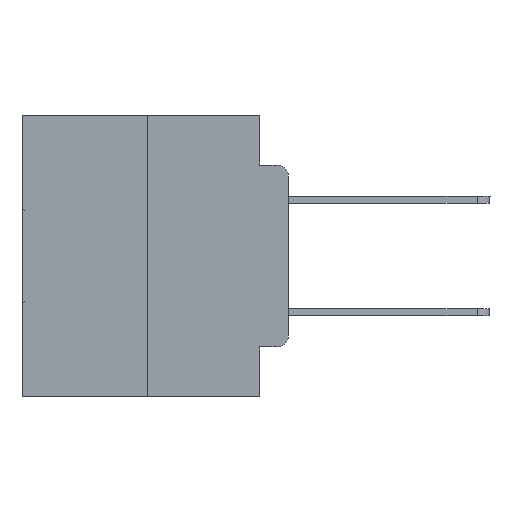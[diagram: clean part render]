
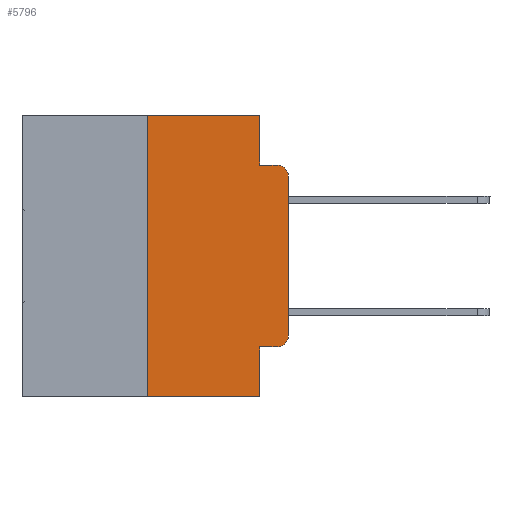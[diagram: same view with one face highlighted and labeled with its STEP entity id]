
A CAD part, left-side view. The second image highlights one B-rep face of the part: STEP entity #5796.
In plain terms, the highlighted planar face has unit normal (-1, 0, 0).
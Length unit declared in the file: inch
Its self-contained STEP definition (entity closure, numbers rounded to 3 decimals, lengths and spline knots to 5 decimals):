
#1228 = LINE ( 'NONE', #22122, #13435 ) ;
#1275 = CARTESIAN_POINT ( 'NONE',  ( 0., 0.051, -0.4115 ) ) ;
#1352 = DIRECTION ( 'NONE',  ( -1., 0., 0. ) ) ;
#1853 = VECTOR ( 'NONE', #12058, 39.37008 ) ;
#3068 = LINE ( 'NONE', #18056, #27924 ) ;
#3337 = ORIENTED_EDGE ( 'NONE', *, *, #27171, .F. ) ;
#3421 = AXIS2_PLACEMENT_3D ( 'NONE', #15892, #1352, #18319 ) ;
#3536 = DIRECTION ( 'NONE',  ( 0., -1., 0. ) ) ;
#3930 = DIRECTION ( 'NONE',  ( 0., -1., 0. ) ) ;
#3946 = CARTESIAN_POINT ( 'NONE',  ( 0., 0., -0.3915 ) ) ;
#3960 = LINE ( 'NONE', #30755, #26572 ) ;
#3976 = EDGE_CURVE ( 'NONE', #16938, #4100, #16561, .T. ) ;
#4100 = VERTEX_POINT ( 'NONE', #24785 ) ;
#4166 = AXIS2_PLACEMENT_3D ( 'NONE', #12298, #22362, #8027 ) ;
#4301 = CARTESIAN_POINT ( 'NONE',  ( 0., 0.051, -0.5 ) ) ;
#4887 = ORIENTED_EDGE ( 'NONE', *, *, #30881, .T. ) ;
#5540 = PLANE ( 'NONE',  #4166 ) ;
#5641 = EDGE_CURVE ( 'NONE', #4100, #10198, #3960, .T. ) ;
#5796 = ADVANCED_FACE ( 'NONE', ( #29119 ), #5540, .F. ) ;
#6980 = VECTOR ( 'NONE', #19574, 39.37008 ) ;
#7313 = EDGE_CURVE ( 'NONE', #11000, #10198, #14852, .T. ) ;
#7492 = VERTEX_POINT ( 'NONE', #21331 ) ;
#7603 = ORIENTED_EDGE ( 'NONE', *, *, #3976, .F. ) ;
#7668 = CIRCLE ( 'NONE', #25949, 0.02 ) ;
#7752 = LINE ( 'NONE', #17192, #6980 ) ;
#8027 = DIRECTION ( 'NONE',  ( 0., 0., -1. ) ) ;
#8768 = EDGE_CURVE ( 'NONE', #22448, #11916, #16369, .T. ) ;
#9472 = VECTOR ( 'NONE', #16045, 39.37008 ) ;
#9676 = CARTESIAN_POINT ( 'NONE',  ( 0., 0., 0. ) ) ;
#10119 = VERTEX_POINT ( 'NONE', #13116 ) ;
#10131 = EDGE_CURVE ( 'NONE', #10119, #16938, #3068, .T. ) ;
#10198 = VERTEX_POINT ( 'NONE', #25469 ) ;
#11000 = VERTEX_POINT ( 'NONE', #29747 ) ;
#11916 = VERTEX_POINT ( 'NONE', #4301 ) ;
#12058 = DIRECTION ( 'NONE',  ( 0., 0., 1. ) ) ;
#12298 = CARTESIAN_POINT ( 'NONE',  ( 0., 0.473, 0. ) ) ;
#12452 = ORIENTED_EDGE ( 'NONE', *, *, #5641, .F. ) ;
#13116 = CARTESIAN_POINT ( 'NONE',  ( 0., 0.25, 0. ) ) ;
#13325 = EDGE_CURVE ( 'NONE', #7492, #24728, #7668, .T. ) ;
#13435 = VECTOR ( 'NONE', #24535, 39.37008 ) ;
#13607 = CARTESIAN_POINT ( 'NONE',  ( 0., 0.051, -0.4115 ) ) ;
#13748 = EDGE_CURVE ( 'NONE', #24728, #11000, #14777, .T. ) ;
#14398 = CARTESIAN_POINT ( 'NONE',  ( 0., 0.02, -0.3915 ) ) ;
#14777 = LINE ( 'NONE', #9676, #1853 ) ;
#14852 = CIRCLE ( 'NONE', #3421, 0.02 ) ;
#15745 = CARTESIAN_POINT ( 'NONE',  ( 0., 0.051, 0. ) ) ;
#15892 = CARTESIAN_POINT ( 'NONE',  ( 0., 0.02, -0.1085 ) ) ;
#16045 = DIRECTION ( 'NONE',  ( 0., 0., -1. ) ) ;
#16111 = CARTESIAN_POINT ( 'NONE',  ( 0., 0.051, 0. ) ) ;
#16369 = LINE ( 'NONE', #22508, #21995 ) ;
#16561 = LINE ( 'NONE', #16111, #9472 ) ;
#16798 = EDGE_LOOP ( 'NONE', ( #29998, #24460, #12452, #7603, #26714, #21093, #28191, #3337, #4887, #18168 ) ) ;
#16825 = DIRECTION ( 'NONE',  ( 0., 0., -1. ) ) ;
#16938 = VERTEX_POINT ( 'NONE', #15745 ) ;
#17192 = CARTESIAN_POINT ( 'NONE',  ( 0., 0.25, 0. ) ) ;
#18056 = CARTESIAN_POINT ( 'NONE',  ( 0., 0.473, 0. ) ) ;
#18168 = ORIENTED_EDGE ( 'NONE', *, *, #13325, .T. ) ;
#18319 = DIRECTION ( 'NONE',  ( 0., 0., -1. ) ) ;
#19028 = CARTESIAN_POINT ( 'NONE',  ( 0., 0.25, -0.5 ) ) ;
#19574 = DIRECTION ( 'NONE',  ( 0., 0., 1. ) ) ;
#19837 = VERTEX_POINT ( 'NONE', #1275 ) ;
#20094 = DIRECTION ( 'NONE',  ( 0., -1., 0. ) ) ;
#21093 = ORIENTED_EDGE ( 'NONE', *, *, #28740, .F. ) ;
#21331 = CARTESIAN_POINT ( 'NONE',  ( 0., 0.02, -0.4115 ) ) ;
#21995 = VECTOR ( 'NONE', #20094, 39.37008 ) ;
#22122 = CARTESIAN_POINT ( 'NONE',  ( 0., 0.051, 0. ) ) ;
#22362 = DIRECTION ( 'NONE',  ( 1., 0., 0. ) ) ;
#22448 = VERTEX_POINT ( 'NONE', #19028 ) ;
#22508 = CARTESIAN_POINT ( 'NONE',  ( 0., 0.473, -0.5 ) ) ;
#24460 = ORIENTED_EDGE ( 'NONE', *, *, #7313, .T. ) ;
#24535 = DIRECTION ( 'NONE',  ( 0., 0., -1. ) ) ;
#24728 = VERTEX_POINT ( 'NONE', #3946 ) ;
#24785 = CARTESIAN_POINT ( 'NONE',  ( 0., 0.051, -0.0885 ) ) ;
#25212 = VECTOR ( 'NONE', #3930, 39.37008 ) ;
#25469 = CARTESIAN_POINT ( 'NONE',  ( 0., 0.02, -0.0885 ) ) ;
#25949 = AXIS2_PLACEMENT_3D ( 'NONE', #14398, #31049, #16825 ) ;
#25970 = LINE ( 'NONE', #13607, #25212 ) ;
#26033 = DIRECTION ( 'NONE',  ( 0., -1., 0. ) ) ;
#26572 = VECTOR ( 'NONE', #26033, 39.37008 ) ;
#26714 = ORIENTED_EDGE ( 'NONE', *, *, #10131, .F. ) ;
#27171 = EDGE_CURVE ( 'NONE', #19837, #11916, #1228, .T. ) ;
#27924 = VECTOR ( 'NONE', #3536, 39.37008 ) ;
#28191 = ORIENTED_EDGE ( 'NONE', *, *, #8768, .T. ) ;
#28740 = EDGE_CURVE ( 'NONE', #22448, #10119, #7752, .T. ) ;
#29119 = FACE_OUTER_BOUND ( 'NONE', #16798, .T. ) ;
#29747 = CARTESIAN_POINT ( 'NONE',  ( 0., 0., -0.1085 ) ) ;
#29998 = ORIENTED_EDGE ( 'NONE', *, *, #13748, .T. ) ;
#30755 = CARTESIAN_POINT ( 'NONE',  ( 0., 0.051, -0.0885 ) ) ;
#30881 = EDGE_CURVE ( 'NONE', #19837, #7492, #25970, .T. ) ;
#31049 = DIRECTION ( 'NONE',  ( -1., 0., 0. ) ) ;
